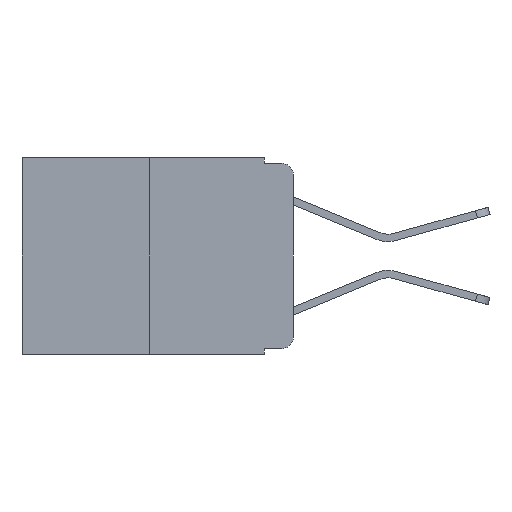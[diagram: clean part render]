
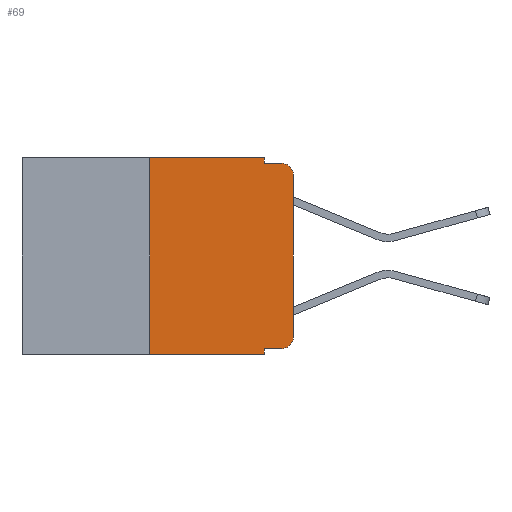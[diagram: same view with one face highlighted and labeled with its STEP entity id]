
A CAD part, left-side view. The second image highlights one B-rep face of the part: STEP entity #69.
In plain terms, the highlighted planar face has unit normal (-1, 0, 0).
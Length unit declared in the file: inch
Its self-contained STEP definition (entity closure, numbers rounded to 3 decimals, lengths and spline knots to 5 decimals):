
#69 = ADVANCED_FACE ( 'NONE', ( #9936 ), #14797, .F. ) ;
#302 = VECTOR ( 'NONE', #10329, 39.37008 ) ;
#1060 = CARTESIAN_POINT ( 'NONE',  ( 0., 0.051, 0. ) ) ;
#1310 = VERTEX_POINT ( 'NONE', #11460 ) ;
#2062 = DIRECTION ( 'NONE',  ( 0., -1., 0. ) ) ;
#3147 = EDGE_CURVE ( 'NONE', #14663, #11307, #3582, .T. ) ;
#3433 = CARTESIAN_POINT ( 'NONE',  ( 0., 0.02, -0.03 ) ) ;
#3546 = CARTESIAN_POINT ( 'NONE',  ( 0., 0.051, -0.333 ) ) ;
#3582 = LINE ( 'NONE', #19304, #13792 ) ;
#3649 = CARTESIAN_POINT ( 'NONE',  ( 0., 0.051, -0.343 ) ) ;
#4139 = CARTESIAN_POINT ( 'NONE',  ( 0., 0.02, -0.01 ) ) ;
#4355 = CARTESIAN_POINT ( 'NONE',  ( 0., 0.051, 0. ) ) ;
#5029 = VECTOR ( 'NONE', #14624, 39.37008 ) ;
#5411 = AXIS2_PLACEMENT_3D ( 'NONE', #3433, #17546, #12280 ) ;
#5549 = EDGE_CURVE ( 'NONE', #12156, #12389, #20879, .T. ) ;
#5896 = CARTESIAN_POINT ( 'NONE',  ( 0., 0.051, 0. ) ) ;
#6401 = VECTOR ( 'NONE', #18480, 39.37008 ) ;
#6867 = CARTESIAN_POINT ( 'NONE',  ( 0., 0.02, -0.333 ) ) ;
#6883 = VERTEX_POINT ( 'NONE', #21475 ) ;
#7728 = ORIENTED_EDGE ( 'NONE', *, *, #3147, .F. ) ;
#8573 = LINE ( 'NONE', #17456, #302 ) ;
#8677 = CARTESIAN_POINT ( 'NONE',  ( 0., 0.02, -0.313 ) ) ;
#8708 = VECTOR ( 'NONE', #22385, 39.37008 ) ;
#8954 = ORIENTED_EDGE ( 'NONE', *, *, #13345, .T. ) ;
#8977 = CARTESIAN_POINT ( 'NONE',  ( 0., 0.473, 0. ) ) ;
#8993 = LINE ( 'NONE', #1060, #8708 ) ;
#9150 = ORIENTED_EDGE ( 'NONE', *, *, #15483, .F. ) ;
#9481 = CIRCLE ( 'NONE', #5411, 0.02 ) ;
#9541 = VECTOR ( 'NONE', #2062, 39.37008 ) ;
#9809 = CARTESIAN_POINT ( 'NONE',  ( 0., 0.473, -0.343 ) ) ;
#9936 = FACE_OUTER_BOUND ( 'NONE', #13634, .T. ) ;
#10083 = ORIENTED_EDGE ( 'NONE', *, *, #22794, .T. ) ;
#10172 = LINE ( 'NONE', #4355, #10462 ) ;
#10329 = DIRECTION ( 'NONE',  ( 0., 0., 1. ) ) ;
#10462 = VECTOR ( 'NONE', #16763, 39.37008 ) ;
#10590 = CARTESIAN_POINT ( 'NONE',  ( 0., 0., -0.03 ) ) ;
#10682 = EDGE_CURVE ( 'NONE', #1310, #13162, #19542, .T. ) ;
#10934 = ORIENTED_EDGE ( 'NONE', *, *, #10682, .F. ) ;
#10953 = CARTESIAN_POINT ( 'NONE',  ( 0., 0.25, -0.343 ) ) ;
#11307 = VERTEX_POINT ( 'NONE', #4139 ) ;
#11460 = CARTESIAN_POINT ( 'NONE',  ( 0., 0.25, 0. ) ) ;
#11645 = AXIS2_PLACEMENT_3D ( 'NONE', #22025, #18378, #14875 ) ;
#12156 = VERTEX_POINT ( 'NONE', #6867 ) ;
#12280 = DIRECTION ( 'NONE',  ( 0., 0., -1. ) ) ;
#12389 = VERTEX_POINT ( 'NONE', #12953 ) ;
#12445 = VERTEX_POINT ( 'NONE', #10953 ) ;
#12487 = ORIENTED_EDGE ( 'NONE', *, *, #5549, .T. ) ;
#12874 = CARTESIAN_POINT ( 'NONE',  ( 0., 0., 0. ) ) ;
#12953 = CARTESIAN_POINT ( 'NONE',  ( 0., 0., -0.313 ) ) ;
#13162 = VERTEX_POINT ( 'NONE', #5896 ) ;
#13313 = LINE ( 'NONE', #9809, #6401 ) ;
#13345 = EDGE_CURVE ( 'NONE', #12445, #19773, #13313, .T. ) ;
#13634 = EDGE_LOOP ( 'NONE', ( #10083, #21081, #7728, #9150, #10934, #22048, #8954, #18492, #21875, #12487 ) ) ;
#13792 = VECTOR ( 'NONE', #22722, 39.37008 ) ;
#14363 = EDGE_CURVE ( 'NONE', #12445, #1310, #8573, .T. ) ;
#14624 = DIRECTION ( 'NONE',  ( 0., 0., 1. ) ) ;
#14663 = VERTEX_POINT ( 'NONE', #18198 ) ;
#14797 = PLANE ( 'NONE',  #11645 ) ;
#14875 = DIRECTION ( 'NONE',  ( 0., 0., -1. ) ) ;
#15338 = VECTOR ( 'NONE', #15881, 39.37008 ) ;
#15483 = EDGE_CURVE ( 'NONE', #13162, #14663, #10172, .T. ) ;
#15809 = DIRECTION ( 'NONE',  ( -1., 0., 0. ) ) ;
#15881 = DIRECTION ( 'NONE',  ( 0., -1., 0. ) ) ;
#16758 = EDGE_CURVE ( 'NONE', #6883, #19773, #8993, .T. ) ;
#16763 = DIRECTION ( 'NONE',  ( 0., 0., -1. ) ) ;
#17425 = EDGE_CURVE ( 'NONE', #6883, #12156, #20056, .T. ) ;
#17456 = CARTESIAN_POINT ( 'NONE',  ( 0., 0.25, 0. ) ) ;
#17546 = DIRECTION ( 'NONE',  ( -1., 0., 0. ) ) ;
#18198 = CARTESIAN_POINT ( 'NONE',  ( 0., 0.051, -0.01 ) ) ;
#18378 = DIRECTION ( 'NONE',  ( 1., 0., 0. ) ) ;
#18480 = DIRECTION ( 'NONE',  ( 0., -1., 0. ) ) ;
#18492 = ORIENTED_EDGE ( 'NONE', *, *, #16758, .F. ) ;
#18659 = EDGE_CURVE ( 'NONE', #20063, #11307, #9481, .T. ) ;
#19128 = LINE ( 'NONE', #12874, #5029 ) ;
#19304 = CARTESIAN_POINT ( 'NONE',  ( 0., 0.051, -0.01 ) ) ;
#19542 = LINE ( 'NONE', #8977, #9541 ) ;
#19773 = VERTEX_POINT ( 'NONE', #3649 ) ;
#20056 = LINE ( 'NONE', #3546, #15338 ) ;
#20063 = VERTEX_POINT ( 'NONE', #10590 ) ;
#20879 = CIRCLE ( 'NONE', #22416, 0.02 ) ;
#21081 = ORIENTED_EDGE ( 'NONE', *, *, #18659, .T. ) ;
#21234 = DIRECTION ( 'NONE',  ( 0., 0., -1. ) ) ;
#21475 = CARTESIAN_POINT ( 'NONE',  ( 0., 0.051, -0.333 ) ) ;
#21875 = ORIENTED_EDGE ( 'NONE', *, *, #17425, .T. ) ;
#22025 = CARTESIAN_POINT ( 'NONE',  ( 0., 0.473, 0. ) ) ;
#22048 = ORIENTED_EDGE ( 'NONE', *, *, #14363, .F. ) ;
#22385 = DIRECTION ( 'NONE',  ( 0., 0., -1. ) ) ;
#22416 = AXIS2_PLACEMENT_3D ( 'NONE', #8677, #15809, #21234 ) ;
#22722 = DIRECTION ( 'NONE',  ( 0., -1., 0. ) ) ;
#22794 = EDGE_CURVE ( 'NONE', #12389, #20063, #19128, .T. ) ;
